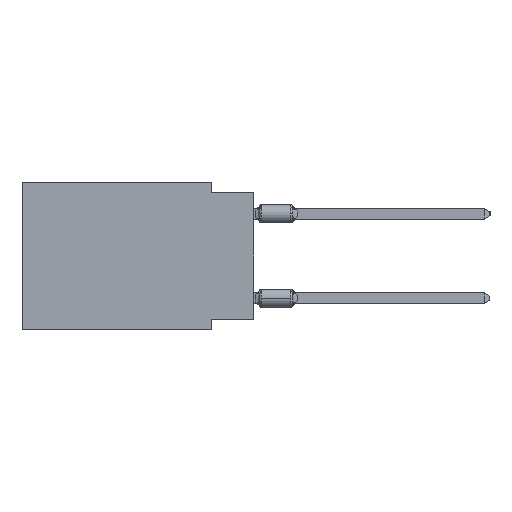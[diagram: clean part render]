
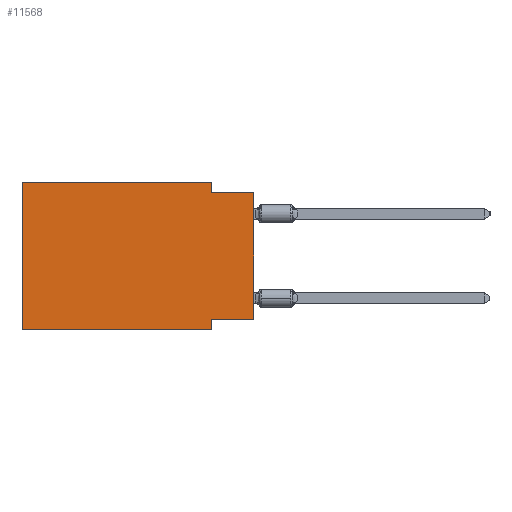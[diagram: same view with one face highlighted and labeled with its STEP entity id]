
A CAD part, left-side view. The second image highlights one B-rep face of the part: STEP entity #11568.
In plain terms, the highlighted planar face has unit normal (-1, 0, 0).
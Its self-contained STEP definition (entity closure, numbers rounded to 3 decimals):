
#22 = CARTESIAN_POINT ( 'NONE',  ( 0., 0., -8.255 ) ) ;
#1787 = ORIENTED_EDGE ( 'NONE', *, *, #27177, .T. ) ;
#1788 = DIRECTION ( 'NONE',  ( 0., -1., 0. ) ) ;
#4471 = LINE ( 'NONE', #16761, #37820 ) ;
#4957 = VERTEX_POINT ( 'NONE', #27415 ) ;
#6687 = DIRECTION ( 'NONE',  ( 0., 0., -1. ) ) ;
#7042 = CARTESIAN_POINT ( 'NONE',  ( 0., 2.54, -8.255 ) ) ;
#7477 = LINE ( 'NONE', #22810, #7840 ) ;
#7840 = VECTOR ( 'NONE', #23209, 1000. ) ;
#7920 = LINE ( 'NONE', #17008, #33307 ) ;
#8022 = VERTEX_POINT ( 'NONE', #26718 ) ;
#8171 = DIRECTION ( 'NONE',  ( 0., 0., -1. ) ) ;
#8685 = EDGE_CURVE ( 'NONE', #33521, #26561, #4471, .T. ) ;
#8873 = VERTEX_POINT ( 'NONE', #23810 ) ;
#9698 = DIRECTION ( 'NONE',  ( 0., 0., 1. ) ) ;
#9806 = LINE ( 'NONE', #22112, #19234 ) ;
#10299 = CARTESIAN_POINT ( 'NONE',  ( 0., 13.97, 0. ) ) ;
#10844 = VERTEX_POINT ( 'NONE', #22 ) ;
#10987 = ORIENTED_EDGE ( 'NONE', *, *, #27536, .F. ) ;
#11531 = ORIENTED_EDGE ( 'NONE', *, *, #33023, .F. ) ;
#11568 = ADVANCED_FACE ( 'NONE', ( #32917 ), #26111, .F. ) ;
#11631 = ORIENTED_EDGE ( 'NONE', *, *, #16170, .F. ) ;
#12599 = CARTESIAN_POINT ( 'NONE',  ( 0., 13.97, -8.89 ) ) ;
#13401 = VERTEX_POINT ( 'NONE', #12599 ) ;
#14036 = VECTOR ( 'NONE', #1788, 1000. ) ;
#14052 = DIRECTION ( 'NONE',  ( 0., 1., 0. ) ) ;
#14450 = CARTESIAN_POINT ( 'NONE',  ( 0., 0., -0.635 ) ) ;
#15006 = CARTESIAN_POINT ( 'NONE',  ( 0., 13.97, -8.89 ) ) ;
#15986 = ORIENTED_EDGE ( 'NONE', *, *, #8685, .F. ) ;
#16113 = EDGE_CURVE ( 'NONE', #10844, #33521, #38782, .T. ) ;
#16170 = EDGE_CURVE ( 'NONE', #4957, #33835, #29363, .T. ) ;
#16751 = LINE ( 'NONE', #10299, #32600 ) ;
#16761 = CARTESIAN_POINT ( 'NONE',  ( 0., 2.54, -8.89 ) ) ;
#17008 = CARTESIAN_POINT ( 'NONE',  ( 0., 13.97, 0. ) ) ;
#17974 = ORIENTED_EDGE ( 'NONE', *, *, #26164, .F. ) ;
#19234 = VECTOR ( 'NONE', #31360, 1000. ) ;
#20509 = CARTESIAN_POINT ( 'NONE',  ( 0., 0., -8.255 ) ) ;
#22112 = CARTESIAN_POINT ( 'NONE',  ( 0., 0., 0. ) ) ;
#22358 = CARTESIAN_POINT ( 'NONE',  ( 0., 2.54, -8.89 ) ) ;
#22395 = VECTOR ( 'NONE', #24297, 1000. ) ;
#22810 = CARTESIAN_POINT ( 'NONE',  ( 0., 2.54, 0. ) ) ;
#23209 = DIRECTION ( 'NONE',  ( 0., 0., -1. ) ) ;
#23810 = CARTESIAN_POINT ( 'NONE',  ( 0., 2.54, 0. ) ) ;
#23894 = CARTESIAN_POINT ( 'NONE',  ( 0., 13.97, 0. ) ) ;
#24297 = DIRECTION ( 'NONE',  ( 0., -1., 0. ) ) ;
#25914 = ORIENTED_EDGE ( 'NONE', *, *, #28212, .T. ) ;
#26111 = PLANE ( 'NONE',  #38057 ) ;
#26164 = EDGE_CURVE ( 'NONE', #13401, #8022, #16751, .T. ) ;
#26561 = VERTEX_POINT ( 'NONE', #22358 ) ;
#26718 = CARTESIAN_POINT ( 'NONE',  ( 0., 13.97, 0. ) ) ;
#27177 = EDGE_CURVE ( 'NONE', #13401, #26561, #33112, .T. ) ;
#27415 = CARTESIAN_POINT ( 'NONE',  ( 0., 2.54, -0.635 ) ) ;
#27536 = EDGE_CURVE ( 'NONE', #8022, #8873, #7920, .T. ) ;
#28212 = EDGE_CURVE ( 'NONE', #10844, #33835, #9806, .T. ) ;
#29363 = LINE ( 'NONE', #14450, #14036 ) ;
#29497 = DIRECTION ( 'NONE',  ( 0., -1., 0. ) ) ;
#31360 = DIRECTION ( 'NONE',  ( 0., 0., 1. ) ) ;
#31776 = ORIENTED_EDGE ( 'NONE', *, *, #16113, .F. ) ;
#32141 = CARTESIAN_POINT ( 'NONE',  ( 0., 0., -0.635 ) ) ;
#32325 = DIRECTION ( 'NONE',  ( 1., 0., 0. ) ) ;
#32600 = VECTOR ( 'NONE', #9698, 1000. ) ;
#32917 = FACE_OUTER_BOUND ( 'NONE', #35894, .T. ) ;
#33023 = EDGE_CURVE ( 'NONE', #8873, #4957, #7477, .T. ) ;
#33112 = LINE ( 'NONE', #15006, #22395 ) ;
#33307 = VECTOR ( 'NONE', #29497, 1000. ) ;
#33521 = VERTEX_POINT ( 'NONE', #7042 ) ;
#33835 = VERTEX_POINT ( 'NONE', #32141 ) ;
#35207 = VECTOR ( 'NONE', #14052, 1000. ) ;
#35894 = EDGE_LOOP ( 'NONE', ( #25914, #11631, #11531, #10987, #17974, #1787, #15986, #31776 ) ) ;
#37820 = VECTOR ( 'NONE', #6687, 1000. ) ;
#38057 = AXIS2_PLACEMENT_3D ( 'NONE', #23894, #32325, #8171 ) ;
#38782 = LINE ( 'NONE', #20509, #35207 ) ;
